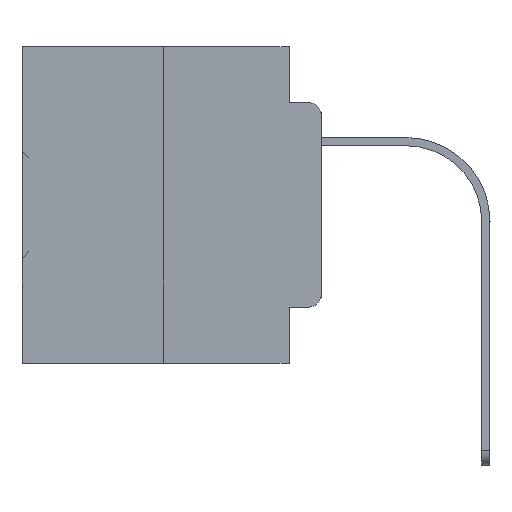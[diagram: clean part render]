
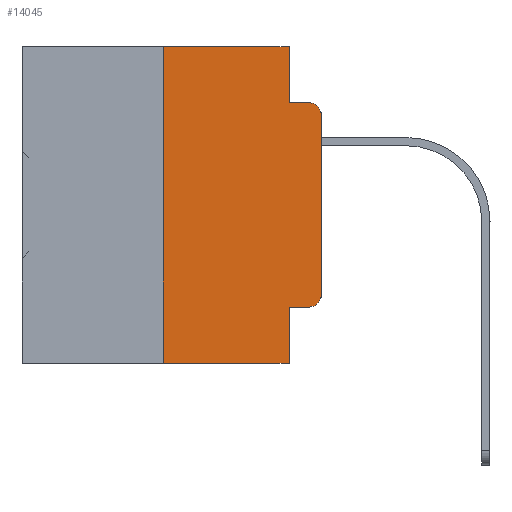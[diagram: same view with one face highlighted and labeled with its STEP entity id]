
A CAD part, left-side view. The second image highlights one B-rep face of the part: STEP entity #14045.
In plain terms, the highlighted planar face has unit normal (-1, 0, 0).
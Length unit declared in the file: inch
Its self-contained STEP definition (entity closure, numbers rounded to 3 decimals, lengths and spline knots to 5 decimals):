
#351 = DIRECTION ( 'NONE',  ( 0., 0., 1. ) ) ;
#469 = EDGE_CURVE ( 'NONE', #26645, #18078, #33394, .T. ) ;
#535 = ORIENTED_EDGE ( 'NONE', *, *, #6087, .F. ) ;
#1874 = CARTESIAN_POINT ( 'NONE',  ( 0., 0.051, -0.0885 ) ) ;
#3582 = CARTESIAN_POINT ( 'NONE',  ( 0., 0.02, -0.0885 ) ) ;
#3894 = ORIENTED_EDGE ( 'NONE', *, *, #30882, .T. ) ;
#4659 = LINE ( 'NONE', #36777, #22516 ) ;
#5321 = EDGE_CURVE ( 'NONE', #9527, #27798, #27277, .T. ) ;
#5542 = EDGE_LOOP ( 'NONE', ( #11120, #29519, #535, #12252, #28251, #18343, #3894, #25971, #11534, #18564 ) ) ;
#6087 = EDGE_CURVE ( 'NONE', #29385, #27798, #15198, .T. ) ;
#6422 = CARTESIAN_POINT ( 'NONE',  ( 0., 0.02, -0.1085 ) ) ;
#6522 = CARTESIAN_POINT ( 'NONE',  ( 0., 0.051, -0.0885 ) ) ;
#6612 = CARTESIAN_POINT ( 'NONE',  ( 0., 0., -0.1085 ) ) ;
#6890 = DIRECTION ( 'NONE',  ( 0., 0., 1. ) ) ;
#7177 = LINE ( 'NONE', #25450, #27458 ) ;
#7619 = VECTOR ( 'NONE', #351, 39.37008 ) ;
#9161 = DIRECTION ( 'NONE',  ( 1., 0., 0. ) ) ;
#9527 = VERTEX_POINT ( 'NONE', #6612 ) ;
#9655 = CARTESIAN_POINT ( 'NONE',  ( 0., 0.051, 0. ) ) ;
#9723 = EDGE_CURVE ( 'NONE', #9905, #26645, #7177, .T. ) ;
#9905 = VERTEX_POINT ( 'NONE', #30019 ) ;
#11120 = ORIENTED_EDGE ( 'NONE', *, *, #29270, .T. ) ;
#11201 = EDGE_CURVE ( 'NONE', #17830, #29385, #36191, .T. ) ;
#11428 = CARTESIAN_POINT ( 'NONE',  ( 0., 0.051, -0.5 ) ) ;
#11534 = ORIENTED_EDGE ( 'NONE', *, *, #9723, .T. ) ;
#12047 = FACE_OUTER_BOUND ( 'NONE', #5542, .T. ) ;
#12252 = ORIENTED_EDGE ( 'NONE', *, *, #11201, .F. ) ;
#12550 = CARTESIAN_POINT ( 'NONE',  ( 0., 0.051, 0. ) ) ;
#12588 = DIRECTION ( 'NONE',  ( 0., 0., -1. ) ) ;
#12689 = LINE ( 'NONE', #21162, #20577 ) ;
#13101 = VECTOR ( 'NONE', #29836, 39.37008 ) ;
#13544 = DIRECTION ( 'NONE',  ( 0., -1., 0. ) ) ;
#14045 = ADVANCED_FACE ( 'NONE', ( #12047 ), #35490, .F. ) ;
#14443 = VECTOR ( 'NONE', #31452, 39.37008 ) ;
#14715 = DIRECTION ( 'NONE',  ( 0., 0., -1. ) ) ;
#15133 = DIRECTION ( 'NONE',  ( 0., 0., -1. ) ) ;
#15198 = LINE ( 'NONE', #6522, #26787 ) ;
#15509 = VERTEX_POINT ( 'NONE', #11428 ) ;
#15554 = AXIS2_PLACEMENT_3D ( 'NONE', #6422, #18169, #12588 ) ;
#15716 = EDGE_CURVE ( 'NONE', #9905, #15509, #4659, .T. ) ;
#17830 = VERTEX_POINT ( 'NONE', #9655 ) ;
#17861 = LINE ( 'NONE', #29556, #32801 ) ;
#17896 = LINE ( 'NONE', #26718, #7619 ) ;
#18078 = VERTEX_POINT ( 'NONE', #22908 ) ;
#18114 = AXIS2_PLACEMENT_3D ( 'NONE', #29336, #9161, #15133 ) ;
#18169 = DIRECTION ( 'NONE',  ( -1., 0., 0. ) ) ;
#18343 = ORIENTED_EDGE ( 'NONE', *, *, #29033, .F. ) ;
#18435 = VERTEX_POINT ( 'NONE', #23251 ) ;
#18564 = ORIENTED_EDGE ( 'NONE', *, *, #469, .T. ) ;
#20577 = VECTOR ( 'NONE', #6890, 39.37008 ) ;
#20671 = CARTESIAN_POINT ( 'NONE',  ( 0., 0.02, -0.3915 ) ) ;
#21162 = CARTESIAN_POINT ( 'NONE',  ( 0., 0., 0. ) ) ;
#22516 = VECTOR ( 'NONE', #25625, 39.37008 ) ;
#22908 = CARTESIAN_POINT ( 'NONE',  ( 0., 0., -0.3915 ) ) ;
#23251 = CARTESIAN_POINT ( 'NONE',  ( 0., 0.25, 0. ) ) ;
#23812 = DIRECTION ( 'NONE',  ( 0., -1., 0. ) ) ;
#25450 = CARTESIAN_POINT ( 'NONE',  ( 0., 0.051, -0.4115 ) ) ;
#25625 = DIRECTION ( 'NONE',  ( 0., 0., -1. ) ) ;
#25971 = ORIENTED_EDGE ( 'NONE', *, *, #15716, .F. ) ;
#26645 = VERTEX_POINT ( 'NONE', #33515 ) ;
#26718 = CARTESIAN_POINT ( 'NONE',  ( 0., 0.25, 0. ) ) ;
#26787 = VECTOR ( 'NONE', #29970, 39.37008 ) ;
#27277 = CIRCLE ( 'NONE', #15554, 0.02 ) ;
#27458 = VECTOR ( 'NONE', #13544, 39.37008 ) ;
#27798 = VERTEX_POINT ( 'NONE', #3582 ) ;
#28251 = ORIENTED_EDGE ( 'NONE', *, *, #31107, .F. ) ;
#29033 = EDGE_CURVE ( 'NONE', #31977, #18435, #17896, .T. ) ;
#29270 = EDGE_CURVE ( 'NONE', #18078, #9527, #12689, .T. ) ;
#29336 = CARTESIAN_POINT ( 'NONE',  ( 0., 0.473, 0. ) ) ;
#29385 = VERTEX_POINT ( 'NONE', #1874 ) ;
#29519 = ORIENTED_EDGE ( 'NONE', *, *, #5321, .T. ) ;
#29556 = CARTESIAN_POINT ( 'NONE',  ( 0., 0.473, -0.5 ) ) ;
#29836 = DIRECTION ( 'NONE',  ( 0., 0., -1. ) ) ;
#29858 = DIRECTION ( 'NONE',  ( -1., 0., 0. ) ) ;
#29970 = DIRECTION ( 'NONE',  ( 0., -1., 0. ) ) ;
#30019 = CARTESIAN_POINT ( 'NONE',  ( 0., 0.051, -0.4115 ) ) ;
#30699 = LINE ( 'NONE', #33773, #14443 ) ;
#30882 = EDGE_CURVE ( 'NONE', #31977, #15509, #17861, .T. ) ;
#31107 = EDGE_CURVE ( 'NONE', #18435, #17830, #30699, .T. ) ;
#31329 = CARTESIAN_POINT ( 'NONE',  ( 0., 0.25, -0.5 ) ) ;
#31452 = DIRECTION ( 'NONE',  ( 0., -1., 0. ) ) ;
#31977 = VERTEX_POINT ( 'NONE', #31329 ) ;
#32801 = VECTOR ( 'NONE', #23812, 39.37008 ) ;
#33394 = CIRCLE ( 'NONE', #34626, 0.02 ) ;
#33515 = CARTESIAN_POINT ( 'NONE',  ( 0., 0.02, -0.4115 ) ) ;
#33773 = CARTESIAN_POINT ( 'NONE',  ( 0., 0.473, 0. ) ) ;
#34626 = AXIS2_PLACEMENT_3D ( 'NONE', #20671, #29858, #14715 ) ;
#35490 = PLANE ( 'NONE',  #18114 ) ;
#36191 = LINE ( 'NONE', #12550, #13101 ) ;
#36777 = CARTESIAN_POINT ( 'NONE',  ( 0., 0.051, 0. ) ) ;
